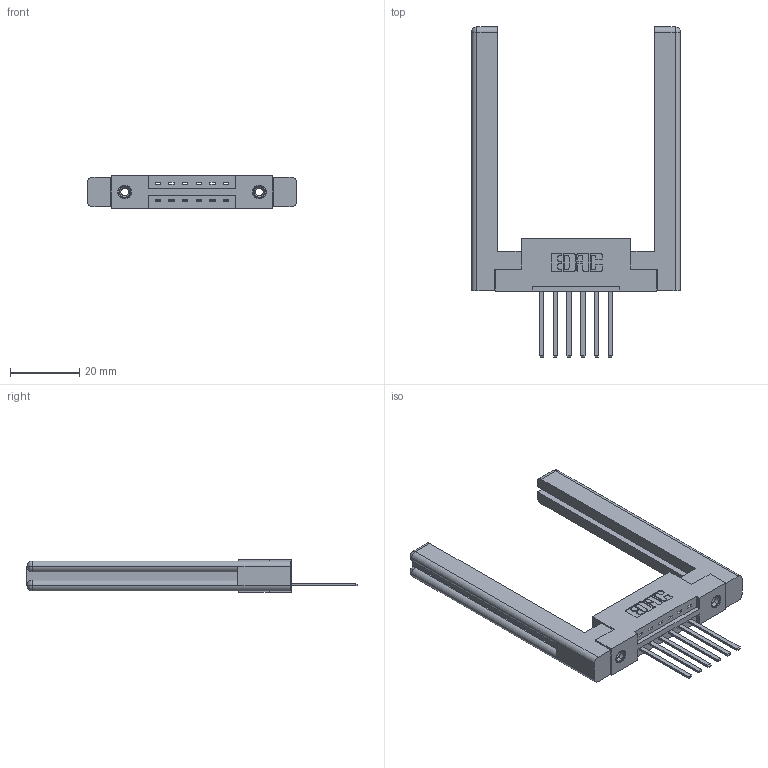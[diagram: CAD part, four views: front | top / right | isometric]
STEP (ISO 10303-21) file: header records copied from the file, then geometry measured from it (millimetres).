
FILE_DESCRIPTION (( 'STEP AP203' ), '1' );
FILE_NAME ('387-006-544-158.STEP', '2019-10-02T01:20:05', ( '' ), ( '' ), 'SwSTEP 2.0', 'SolidWorks 2016', '' );
FILE_SCHEMA (( 'CONFIG_CONTROL_DESIGN' ));
Length unit declared in the file: inch
Products named in the file (5): 345-250-001_345-250-001-102; 307-220-058; 337 Part_Flush Mounting Lugs - 0.156 Dia-TI; 387-006-544-158; 345-292-001_345-293-144
Assembly tree (11 placements, depth 2):
  387-006-544-158
    337 Part_Flush Mounting Lugs - 0.156 Dia-TI
    345-292-001_345-293-144  x6
    345-250-001_345-250-001-102  x2
    307-220-058  x2
Bounding box: 60.4 x 95.38 x 9.4 mm (x, y, z)
Volume: 13058.8 mm3; surface area: 11335.2 mm2
Topology: 11 solids, 11 shells, 592 faces, 1685 edges, 1102 vertices
Faces by surface type: plane 406, cylinder 162, cone 12, torus 12
Entity records: 11566 total; most frequent: CARTESIAN_POINT 2011, ORIENTED_EDGE 1892, DIRECTION 1782, EDGE_CURVE 946, LINE 774, VECTOR 774, VERTEX_POINT 622, AXIS2_PLACEMENT_3D 504
